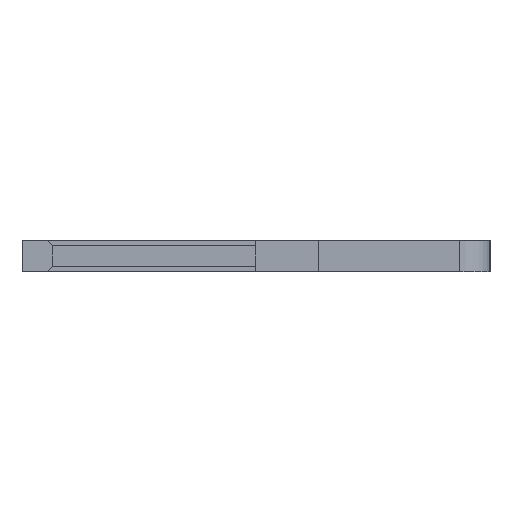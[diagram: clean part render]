
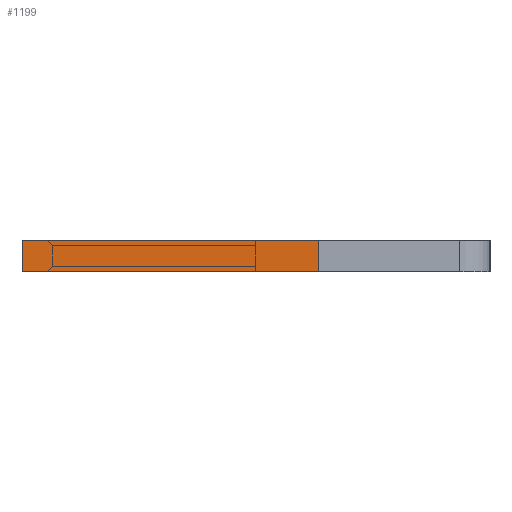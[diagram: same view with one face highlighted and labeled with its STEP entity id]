
A CAD part, left-side view. The second image highlights one B-rep face of the part: STEP entity #1199.
In plain terms, the highlighted face is planar.
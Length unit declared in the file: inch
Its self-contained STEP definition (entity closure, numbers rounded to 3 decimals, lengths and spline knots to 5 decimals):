
#4 = AXIS2_PLACEMENT_3D ( 'NONE', #141, #195, #699 ) ;
#54 = EDGE_CURVE ( 'NONE', #686, #1755, #884, .T. ) ;
#103 = LINE ( 'NONE', #1701, #2261 ) ;
#135 = VECTOR ( 'NONE', #1509, 39.37008 ) ;
#141 = CARTESIAN_POINT ( 'NONE',  ( 0.01, 0.15, -0.04 ) ) ;
#195 = DIRECTION ( 'NONE',  ( 0., 0., 1. ) ) ;
#202 = VERTEX_POINT ( 'NONE', #2154 ) ;
#227 = LINE ( 'NONE', #1915, #135 ) ;
#496 = ORIENTED_EDGE ( 'NONE', *, *, #2312, .T. ) ;
#531 = ORIENTED_EDGE ( 'NONE', *, *, #54, .T. ) ;
#577 = DIRECTION ( 'NONE',  ( 0., 1., 0. ) ) ;
#584 = VECTOR ( 'NONE', #577, 39.37008 ) ;
#647 = VECTOR ( 'NONE', #1086, 39.37008 ) ;
#686 = VERTEX_POINT ( 'NONE', #2229 ) ;
#699 = DIRECTION ( 'NONE',  ( 1., 0., 0. ) ) ;
#884 = LINE ( 'NONE', #1721, #647 ) ;
#1030 = VERTEX_POINT ( 'NONE', #1594 ) ;
#1072 = EDGE_CURVE ( 'NONE', #1030, #202, #1137, .T. ) ;
#1086 = DIRECTION ( 'NONE',  ( 0., 1., 0. ) ) ;
#1137 = LINE ( 'NONE', #1983, #584 ) ;
#1199 = ADVANCED_FACE ( 'NONE', ( #1380 ), #2421, .F. ) ;
#1380 = FACE_OUTER_BOUND ( 'NONE', #2298, .T. ) ;
#1509 = DIRECTION ( 'NONE',  ( -1., 0., 0. ) ) ;
#1594 = CARTESIAN_POINT ( 'NONE',  ( 0.01, -0.04, -0.04 ) ) ;
#1701 = CARTESIAN_POINT ( 'NONE',  ( 0.01, 0.15, -0.04 ) ) ;
#1721 = CARTESIAN_POINT ( 'NONE',  ( -0.01, 0.15, -0.04 ) ) ;
#1755 = VERTEX_POINT ( 'NONE', #2097 ) ;
#1792 = EDGE_CURVE ( 'NONE', #202, #1755, #103, .T. ) ;
#1813 = ORIENTED_EDGE ( 'NONE', *, *, #1792, .F. ) ;
#1915 = CARTESIAN_POINT ( 'NONE',  ( 0.01, -0.04, -0.04 ) ) ;
#1983 = CARTESIAN_POINT ( 'NONE',  ( 0.01, 0.15, -0.04 ) ) ;
#2060 = ORIENTED_EDGE ( 'NONE', *, *, #1072, .F. ) ;
#2070 = DIRECTION ( 'NONE',  ( -1., 0., 0. ) ) ;
#2097 = CARTESIAN_POINT ( 'NONE',  ( -0.01, 0.15, -0.04 ) ) ;
#2154 = CARTESIAN_POINT ( 'NONE',  ( 0.01, 0.15, -0.04 ) ) ;
#2229 = CARTESIAN_POINT ( 'NONE',  ( -0.01, -0.04, -0.04 ) ) ;
#2261 = VECTOR ( 'NONE', #2070, 39.37008 ) ;
#2298 = EDGE_LOOP ( 'NONE', ( #531, #1813, #2060, #496 ) ) ;
#2312 = EDGE_CURVE ( 'NONE', #1030, #686, #227, .T. ) ;
#2421 = PLANE ( 'NONE',  #4 ) ;
